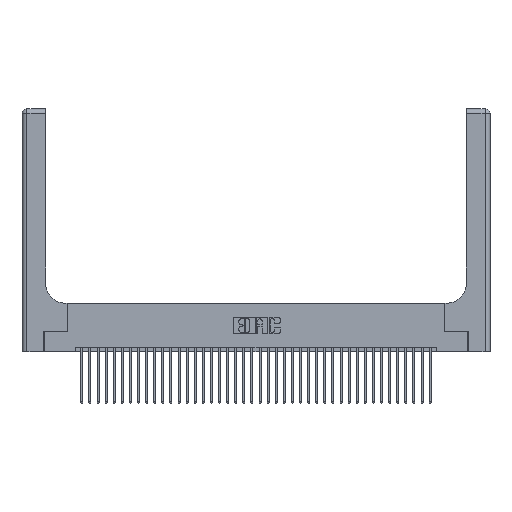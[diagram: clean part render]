
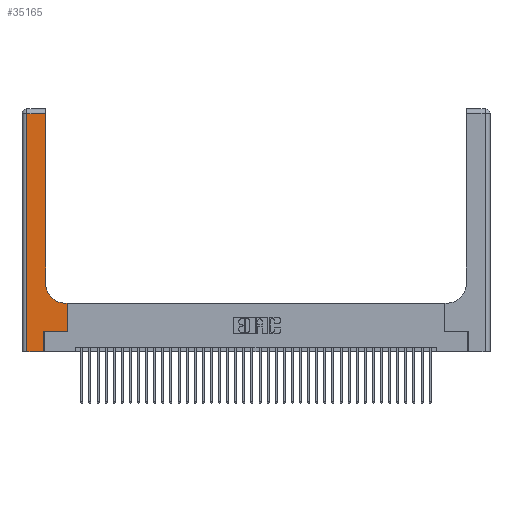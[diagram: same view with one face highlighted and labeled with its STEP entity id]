
A CAD part, top view. The second image highlights one B-rep face of the part: STEP entity #35165.
In plain terms, the highlighted planar face has unit normal (0, 0, 1).
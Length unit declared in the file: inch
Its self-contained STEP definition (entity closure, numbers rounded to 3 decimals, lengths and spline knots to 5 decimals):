
#1307 = CARTESIAN_POINT ( 'NONE',  ( 0., 0., 0.37 ) ) ;
#1320 = CARTESIAN_POINT ( 'NONE',  ( 0.06, 0., 0.37 ) ) ;
#1729 = VERTEX_POINT ( 'NONE', #23873 ) ;
#1793 = CARTESIAN_POINT ( 'NONE',  ( 0., 3., 0.37 ) ) ;
#2404 = CARTESIAN_POINT ( 'NONE',  ( 0.5415, 0.85, 0.37 ) ) ;
#3489 = VERTEX_POINT ( 'NONE', #1320 ) ;
#3606 = ORIENTED_EDGE ( 'NONE', *, *, #33439, .T. ) ;
#3715 = CARTESIAN_POINT ( 'NONE',  ( 0.269, 0.25, 0.37 ) ) ;
#3970 = CARTESIAN_POINT ( 'NONE',  ( 0.5585, 0.25, 0.37 ) ) ;
#4954 = DIRECTION ( 'NONE',  ( -1., 0., 0. ) ) ;
#5557 = ORIENTED_EDGE ( 'NONE', *, *, #20143, .T. ) ;
#5572 = DIRECTION ( 'NONE',  ( 1., 0., 0. ) ) ;
#5609 = VERTEX_POINT ( 'NONE', #36008 ) ;
#7262 = DIRECTION ( 'NONE',  ( 0., 1., 0. ) ) ;
#7290 = ORIENTED_EDGE ( 'NONE', *, *, #11872, .T. ) ;
#7572 = VECTOR ( 'NONE', #27555, 39.37008 ) ;
#7848 = EDGE_CURVE ( 'NONE', #36450, #19683, #21016, .T. ) ;
#9229 = CARTESIAN_POINT ( 'NONE',  ( 0., 2.94, 0.37 ) ) ;
#10335 = CARTESIAN_POINT ( 'NONE',  ( 0.06, 3., 0.37 ) ) ;
#11035 = DIRECTION ( 'NONE',  ( -1., 0., 0. ) ) ;
#11244 = LINE ( 'NONE', #14656, #34438 ) ;
#11872 = EDGE_CURVE ( 'NONE', #1729, #28343, #23768, .T. ) ;
#12683 = ORIENTED_EDGE ( 'NONE', *, *, #22640, .T. ) ;
#12876 = VECTOR ( 'NONE', #11035, 39.37008 ) ;
#13409 = DIRECTION ( 'NONE',  ( 0., -1., 0. ) ) ;
#14475 = LINE ( 'NONE', #1307, #23482 ) ;
#14656 = CARTESIAN_POINT ( 'NONE',  ( 0.269, 0., 0.37 ) ) ;
#15771 = EDGE_CURVE ( 'NONE', #16094, #36450, #22538, .T. ) ;
#16094 = VERTEX_POINT ( 'NONE', #21554 ) ;
#17145 = ORIENTED_EDGE ( 'NONE', *, *, #7848, .T. ) ;
#19048 = EDGE_CURVE ( 'NONE', #3489, #37598, #14475, .T. ) ;
#19683 = VERTEX_POINT ( 'NONE', #35003 ) ;
#19794 = DIRECTION ( 'NONE',  ( 1., 0., 0. ) ) ;
#20043 = VECTOR ( 'NONE', #39165, 39.37008 ) ;
#20143 = EDGE_CURVE ( 'NONE', #28343, #3489, #24399, .T. ) ;
#20269 = PLANE ( 'NONE',  #24061 ) ;
#20673 = VECTOR ( 'NONE', #7262, 39.37008 ) ;
#20741 = ORIENTED_EDGE ( 'NONE', *, *, #19048, .T. ) ;
#21016 = LINE ( 'NONE', #28011, #12876 ) ;
#21554 = CARTESIAN_POINT ( 'NONE',  ( 0.5585, 0.25, 0.37 ) ) ;
#22538 = LINE ( 'NONE', #3970, #20673 ) ;
#22640 = EDGE_CURVE ( 'NONE', #5609, #16094, #35318, .T. ) ;
#23288 = DIRECTION ( 'NONE',  ( 0., 0., -1. ) ) ;
#23482 = VECTOR ( 'NONE', #19794, 39.37008 ) ;
#23768 = LINE ( 'NONE', #9229, #7572 ) ;
#23862 = DIRECTION ( 'NONE',  ( 0., 0., -1. ) ) ;
#23873 = CARTESIAN_POINT ( 'NONE',  ( 0.2915, 2.94, 0.37 ) ) ;
#24050 = CARTESIAN_POINT ( 'NONE',  ( 0.2915, 3., 0.37 ) ) ;
#24061 = AXIS2_PLACEMENT_3D ( 'NONE', #1793, #23288, #4954 ) ;
#24399 = LINE ( 'NONE', #10335, #31438 ) ;
#25062 = CARTESIAN_POINT ( 'NONE',  ( 0.2915, 0.85, 0.37 ) ) ;
#27555 = DIRECTION ( 'NONE',  ( -1., 0., 0. ) ) ;
#27961 = ORIENTED_EDGE ( 'NONE', *, *, #30254, .T. ) ;
#27968 = CARTESIAN_POINT ( 'NONE',  ( 0.269, 0., 0.37 ) ) ;
#28011 = CARTESIAN_POINT ( 'NONE',  ( 0.2915, 0.6, 0.37 ) ) ;
#28033 = LINE ( 'NONE', #24050, #20043 ) ;
#28145 = DIRECTION ( 'NONE',  ( 1., 0., 0. ) ) ;
#28343 = VERTEX_POINT ( 'NONE', #34906 ) ;
#29345 = VERTEX_POINT ( 'NONE', #25062 ) ;
#29994 = EDGE_LOOP ( 'NONE', ( #3606, #7290, #5557, #20741, #34795, #12683, #39140, #17145, #27961 ) ) ;
#30175 = CIRCLE ( 'NONE', #30500, 0.25 ) ;
#30254 = EDGE_CURVE ( 'NONE', #19683, #29345, #30175, .T. ) ;
#30500 = AXIS2_PLACEMENT_3D ( 'NONE', #2404, #23862, #5572 ) ;
#31072 = CARTESIAN_POINT ( 'NONE',  ( 0.5585, 0.6, 0.37 ) ) ;
#31438 = VECTOR ( 'NONE', #13409, 39.37008 ) ;
#33415 = VECTOR ( 'NONE', #28145, 39.37008 ) ;
#33439 = EDGE_CURVE ( 'NONE', #29345, #1729, #28033, .T. ) ;
#34438 = VECTOR ( 'NONE', #35766, 39.37008 ) ;
#34795 = ORIENTED_EDGE ( 'NONE', *, *, #37332, .T. ) ;
#34906 = CARTESIAN_POINT ( 'NONE',  ( 0.06, 2.94, 0.37 ) ) ;
#35003 = CARTESIAN_POINT ( 'NONE',  ( 0.5415, 0.6, 0.37 ) ) ;
#35165 = ADVANCED_FACE ( 'NONE', ( #36972 ), #20269, .F. ) ;
#35318 = LINE ( 'NONE', #3715, #33415 ) ;
#35766 = DIRECTION ( 'NONE',  ( 0., 1., 0. ) ) ;
#36008 = CARTESIAN_POINT ( 'NONE',  ( 0.269, 0.25, 0.37 ) ) ;
#36450 = VERTEX_POINT ( 'NONE', #31072 ) ;
#36972 = FACE_OUTER_BOUND ( 'NONE', #29994, .T. ) ;
#37332 = EDGE_CURVE ( 'NONE', #37598, #5609, #11244, .T. ) ;
#37598 = VERTEX_POINT ( 'NONE', #27968 ) ;
#39140 = ORIENTED_EDGE ( 'NONE', *, *, #15771, .T. ) ;
#39165 = DIRECTION ( 'NONE',  ( 0., 1., 0. ) ) ;
